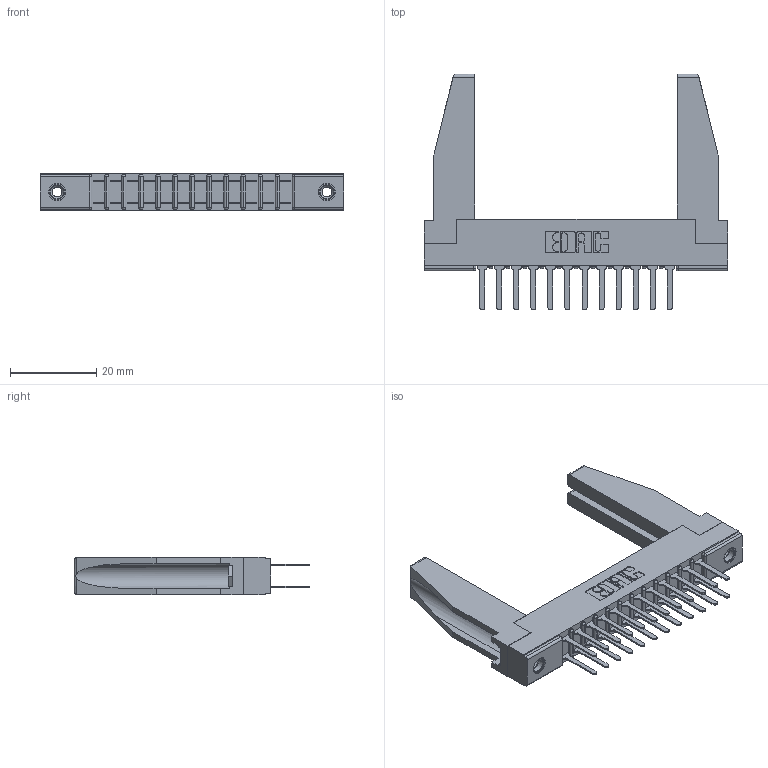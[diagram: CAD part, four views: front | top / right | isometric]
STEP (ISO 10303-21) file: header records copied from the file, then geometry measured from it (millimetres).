
FILE_DESCRIPTION (( 'STEP AP203' ), '1' );
FILE_NAME ('357-024-422-278.STEP', '2020-10-03T00:43:20', ( '' ), ( '' ), 'SwSTEP 2.0', 'SolidWorks 2020', '' );
FILE_SCHEMA (( 'CONFIG_CONTROL_DESIGN' ));
Length unit declared in the file: inch
Products named in the file (5): 357-024-422-278; 307 Part_.156 Dia Mounting Holes; 307-290-001_522; 307-220-078; 345-250-001_345-250-001-102
Assembly tree (29 placements, depth 2):
  357-024-422-278
    307 Part_.156 Dia Mounting Holes
    307-290-001_522  x24
    307-220-078  x2
    345-250-001_345-250-001-102  x2
Bounding box: 70.56 x 54.81 x 8.71 mm (x, y, z)
Volume: 8661.6 mm3; surface area: 11818.4 mm2
Topology: 29 solids, 29 shells, 1365 faces, 3773 edges, 2438 vertices
Faces by surface type: plane 898, cylinder 425, sphere 26, cone 12, torus 4
Entity records: 16777 total; most frequent: CARTESIAN_POINT 2762, ORIENTED_EDGE 2692, DIRECTION 2672, EDGE_CURVE 1346, LINE 1024, VECTOR 1024, VERTEX_POINT 872, AXIS2_PLACEMENT_3D 824
